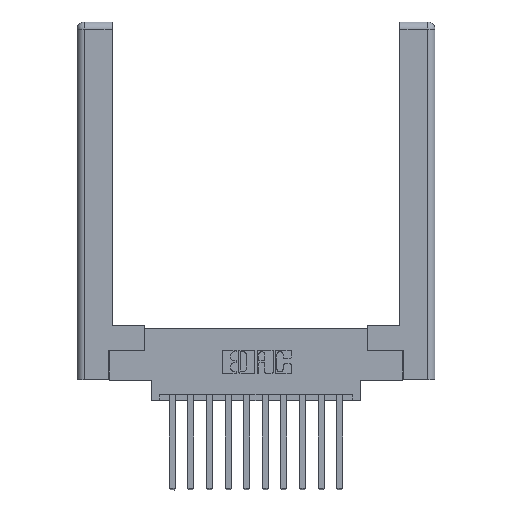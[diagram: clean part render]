
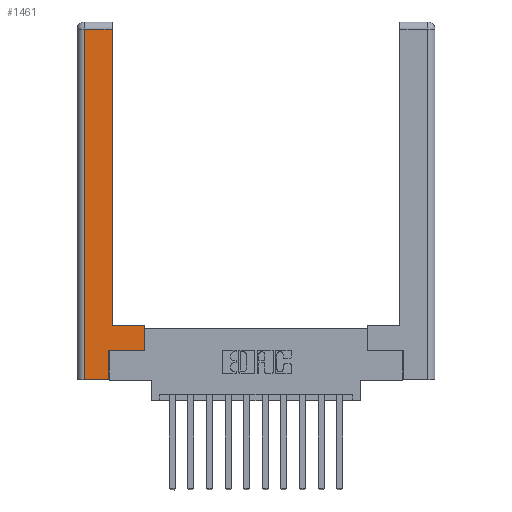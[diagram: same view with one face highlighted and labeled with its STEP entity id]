
A CAD part, top view. The second image highlights one B-rep face of the part: STEP entity #1461.
In plain terms, the highlighted planar face has unit normal (0, 0, 1).
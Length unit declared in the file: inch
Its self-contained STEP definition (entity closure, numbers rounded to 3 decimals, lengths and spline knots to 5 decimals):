
#418 = ORIENTED_EDGE ( 'NONE', *, *, #7871, .T. ) ;
#443 = DIRECTION ( 'NONE',  ( 1., 0., 0. ) ) ;
#656 = DIRECTION ( 'NONE',  ( 0., 0., -1. ) ) ;
#751 = VERTEX_POINT ( 'NONE', #1884 ) ;
#1461 = ADVANCED_FACE ( 'NONE', ( #3906 ), #4160, .F. ) ;
#1803 = CARTESIAN_POINT ( 'NONE',  ( 0.265, 0.245, 0. ) ) ;
#1884 = CARTESIAN_POINT ( 'NONE',  ( 0.0615, 0., 0. ) ) ;
#2040 = EDGE_LOOP ( 'NONE', ( #5058, #3042, #10236, #8123, #418, #14383, #11068, #3708 ) ) ;
#2261 = EDGE_CURVE ( 'NONE', #8020, #751, #9300, .T. ) ;
#2671 = EDGE_CURVE ( 'NONE', #751, #5845, #3018, .T. ) ;
#3015 = CARTESIAN_POINT ( 'NONE',  ( 0.295, 2.94, 0. ) ) ;
#3018 = LINE ( 'NONE', #5997, #10887 ) ;
#3042 = ORIENTED_EDGE ( 'NONE', *, *, #4058, .T. ) ;
#3498 = CARTESIAN_POINT ( 'NONE',  ( 0.295, 0.45, 0. ) ) ;
#3708 = ORIENTED_EDGE ( 'NONE', *, *, #5068, .T. ) ;
#3906 = FACE_OUTER_BOUND ( 'NONE', #2040, .T. ) ;
#3963 = VECTOR ( 'NONE', #9782, 39.37008 ) ;
#4058 = EDGE_CURVE ( 'NONE', #11880, #8020, #5590, .T. ) ;
#4160 = PLANE ( 'NONE',  #5679 ) ;
#4833 = EDGE_CURVE ( 'NONE', #9952, #11880, #9225, .T. ) ;
#4868 = CARTESIAN_POINT ( 'NONE',  ( 0.565, 0.245, 0. ) ) ;
#4929 = DIRECTION ( 'NONE',  ( 0., 1., 0. ) ) ;
#5058 = ORIENTED_EDGE ( 'NONE', *, *, #4833, .T. ) ;
#5068 = EDGE_CURVE ( 'NONE', #11363, #9952, #7850, .T. ) ;
#5431 = DIRECTION ( 'NONE',  ( -1., 0., 0. ) ) ;
#5474 = CARTESIAN_POINT ( 'NONE',  ( 0.0615, 2.94, 0. ) ) ;
#5590 = LINE ( 'NONE', #6786, #8234 ) ;
#5679 = AXIS2_PLACEMENT_3D ( 'NONE', #9646, #656, #10775 ) ;
#5845 = VERTEX_POINT ( 'NONE', #6174 ) ;
#5942 = LINE ( 'NONE', #12199, #9632 ) ;
#5997 = CARTESIAN_POINT ( 'NONE',  ( 0.265, 0., 0. ) ) ;
#6174 = CARTESIAN_POINT ( 'NONE',  ( 0.265, 0., 0. ) ) ;
#6263 = VERTEX_POINT ( 'NONE', #4868 ) ;
#6327 = CARTESIAN_POINT ( 'NONE',  ( 0.295, 3., 0. ) ) ;
#6432 = CARTESIAN_POINT ( 'NONE',  ( 0.0615, 0., 0. ) ) ;
#6786 = CARTESIAN_POINT ( 'NONE',  ( 0.0615, 2.94, 0. ) ) ;
#7036 = DIRECTION ( 'NONE',  ( -1., 0., 0. ) ) ;
#7850 = LINE ( 'NONE', #3498, #8705 ) ;
#7871 = EDGE_CURVE ( 'NONE', #5845, #8945, #13468, .T. ) ;
#7902 = DIRECTION ( 'NONE',  ( 1., 0., 0. ) ) ;
#8020 = VERTEX_POINT ( 'NONE', #5474 ) ;
#8051 = EDGE_CURVE ( 'NONE', #8945, #6263, #5942, .T. ) ;
#8055 = LINE ( 'NONE', #9591, #8752 ) ;
#8123 = ORIENTED_EDGE ( 'NONE', *, *, #2671, .T. ) ;
#8234 = VECTOR ( 'NONE', #5431, 39.37008 ) ;
#8705 = VECTOR ( 'NONE', #7036, 39.37008 ) ;
#8752 = VECTOR ( 'NONE', #4929, 39.37008 ) ;
#8945 = VERTEX_POINT ( 'NONE', #12487 ) ;
#9225 = LINE ( 'NONE', #6327, #3963 ) ;
#9300 = LINE ( 'NONE', #6432, #14175 ) ;
#9591 = CARTESIAN_POINT ( 'NONE',  ( 0.565, 0.45, 0. ) ) ;
#9632 = VECTOR ( 'NONE', #7902, 39.37008 ) ;
#9641 = DIRECTION ( 'NONE',  ( 0., -1., 0. ) ) ;
#9646 = CARTESIAN_POINT ( 'NONE',  ( 0., 0., 0. ) ) ;
#9782 = DIRECTION ( 'NONE',  ( 0., 1., 0. ) ) ;
#9952 = VERTEX_POINT ( 'NONE', #14275 ) ;
#10236 = ORIENTED_EDGE ( 'NONE', *, *, #2261, .T. ) ;
#10775 = DIRECTION ( 'NONE',  ( -1., 0., 0. ) ) ;
#10887 = VECTOR ( 'NONE', #443, 39.37008 ) ;
#11068 = ORIENTED_EDGE ( 'NONE', *, *, #13550, .T. ) ;
#11363 = VERTEX_POINT ( 'NONE', #13222 ) ;
#11880 = VERTEX_POINT ( 'NONE', #3015 ) ;
#12199 = CARTESIAN_POINT ( 'NONE',  ( 0.565, 0.245, 0. ) ) ;
#12487 = CARTESIAN_POINT ( 'NONE',  ( 0.265, 0.245, 0. ) ) ;
#12906 = DIRECTION ( 'NONE',  ( 0., 1., 0. ) ) ;
#13124 = VECTOR ( 'NONE', #12906, 39.37008 ) ;
#13222 = CARTESIAN_POINT ( 'NONE',  ( 0.565, 0.45, 0. ) ) ;
#13468 = LINE ( 'NONE', #1803, #13124 ) ;
#13550 = EDGE_CURVE ( 'NONE', #6263, #11363, #8055, .T. ) ;
#14175 = VECTOR ( 'NONE', #9641, 39.37008 ) ;
#14275 = CARTESIAN_POINT ( 'NONE',  ( 0.295, 0.45, 0. ) ) ;
#14383 = ORIENTED_EDGE ( 'NONE', *, *, #8051, .T. ) ;
